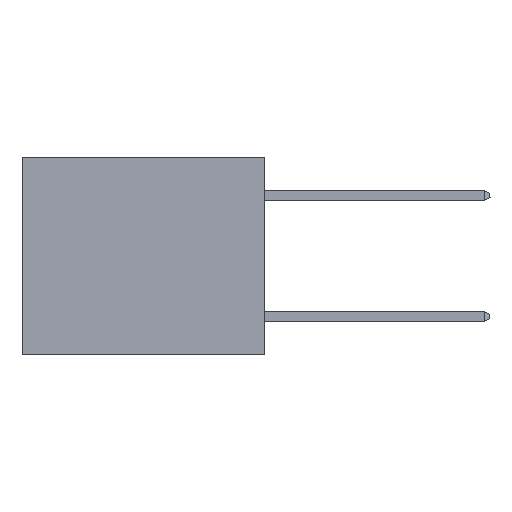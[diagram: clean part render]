
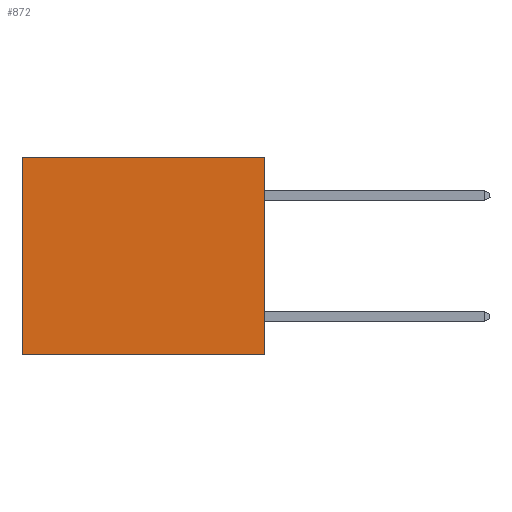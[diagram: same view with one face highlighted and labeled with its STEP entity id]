
A CAD part, left-side view. The second image highlights one B-rep face of the part: STEP entity #872.
In plain terms, the highlighted planar face has unit normal (-1, 0, 0).
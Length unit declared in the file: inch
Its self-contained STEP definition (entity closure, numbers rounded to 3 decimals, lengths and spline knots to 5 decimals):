
#230 = DIRECTION ( 'NONE',  ( 1., 0., 0. ) ) ;
#443 = ORIENTED_EDGE ( 'NONE', *, *, #11925, .F. ) ;
#872 = ADVANCED_FACE ( 'NONE', ( #21572 ), #7074, .F. ) ;
#1153 = VECTOR ( 'NONE', #17417, 39.37008 ) ;
#2904 = CARTESIAN_POINT ( 'NONE',  ( 0.3165, 0.6, -0.49 ) ) ;
#2916 = CARTESIAN_POINT ( 'NONE',  ( 0.3165, 0., -0.49 ) ) ;
#3499 = EDGE_CURVE ( 'NONE', #4311, #16458, #15924, .T. ) ;
#3919 = CARTESIAN_POINT ( 'NONE',  ( 0.3165, 0., 0. ) ) ;
#4286 = LINE ( 'NONE', #2904, #13968 ) ;
#4311 = VERTEX_POINT ( 'NONE', #3919 ) ;
#5426 = VECTOR ( 'NONE', #19367, 39.37008 ) ;
#6409 = LINE ( 'NONE', #15189, #5426 ) ;
#7074 = PLANE ( 'NONE',  #11439 ) ;
#7158 = DIRECTION ( 'NONE',  ( 0., 0., -1. ) ) ;
#8753 = EDGE_CURVE ( 'NONE', #4311, #12855, #6409, .T. ) ;
#8803 = VECTOR ( 'NONE', #17551, 39.37008 ) ;
#9020 = CARTESIAN_POINT ( 'NONE',  ( 0.3165, 0., -0.49 ) ) ;
#11149 = CARTESIAN_POINT ( 'NONE',  ( 0.3165, 0.6, 0. ) ) ;
#11195 = CARTESIAN_POINT ( 'NONE',  ( 0.3165, 0., -0.49 ) ) ;
#11439 = AXIS2_PLACEMENT_3D ( 'NONE', #11195, #230, #7158 ) ;
#11925 = EDGE_CURVE ( 'NONE', #16458, #26566, #16433, .T. ) ;
#12855 = VERTEX_POINT ( 'NONE', #11149 ) ;
#13663 = EDGE_LOOP ( 'NONE', ( #16315, #443, #15381, #24011 ) ) ;
#13968 = VECTOR ( 'NONE', #21304, 39.37008 ) ;
#15189 = CARTESIAN_POINT ( 'NONE',  ( 0.3165, 0., 0. ) ) ;
#15381 = ORIENTED_EDGE ( 'NONE', *, *, #3499, .F. ) ;
#15924 = LINE ( 'NONE', #9020, #8803 ) ;
#16175 = CARTESIAN_POINT ( 'NONE',  ( 0.3165, 0.6, -0.49 ) ) ;
#16315 = ORIENTED_EDGE ( 'NONE', *, *, #24399, .T. ) ;
#16433 = LINE ( 'NONE', #20821, #1153 ) ;
#16458 = VERTEX_POINT ( 'NONE', #2916 ) ;
#17417 = DIRECTION ( 'NONE',  ( 0., 1., 0. ) ) ;
#17551 = DIRECTION ( 'NONE',  ( 0., 0., -1. ) ) ;
#19367 = DIRECTION ( 'NONE',  ( 0., 1., 0. ) ) ;
#20821 = CARTESIAN_POINT ( 'NONE',  ( 0.3165, 0., -0.49 ) ) ;
#21304 = DIRECTION ( 'NONE',  ( 0., 0., -1. ) ) ;
#21572 = FACE_OUTER_BOUND ( 'NONE', #13663, .T. ) ;
#24011 = ORIENTED_EDGE ( 'NONE', *, *, #8753, .T. ) ;
#24399 = EDGE_CURVE ( 'NONE', #12855, #26566, #4286, .T. ) ;
#26566 = VERTEX_POINT ( 'NONE', #16175 ) ;
